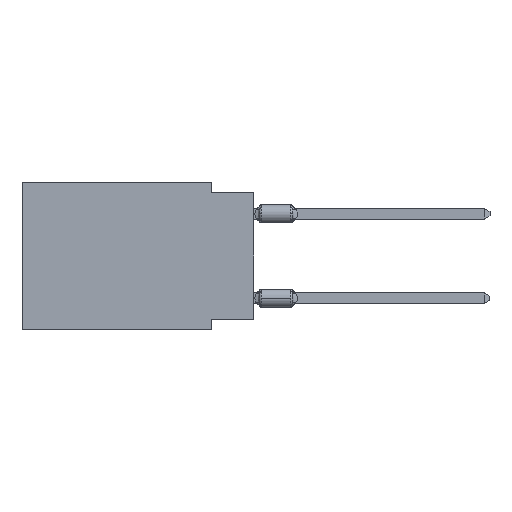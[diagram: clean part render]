
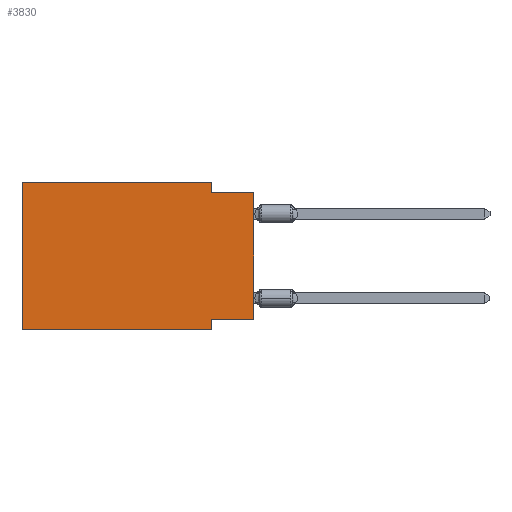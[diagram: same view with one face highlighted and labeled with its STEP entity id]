
A CAD part, left-side view. The second image highlights one B-rep face of the part: STEP entity #3830.
In plain terms, the highlighted planar face has unit normal (-1, 0, 0).
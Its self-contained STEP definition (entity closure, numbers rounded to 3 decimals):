
#281 = VERTEX_POINT ( 'NONE', #9532 ) ;
#521 = LINE ( 'NONE', #2627, #18176 ) ;
#1229 = ORIENTED_EDGE ( 'NONE', *, *, #23193, .F. ) ;
#1384 = DIRECTION ( 'NONE',  ( 0., 0., 1. ) ) ;
#1416 = EDGE_CURVE ( 'NONE', #16561, #22516, #3240, .T. ) ;
#1538 = FACE_OUTER_BOUND ( 'NONE', #6726, .T. ) ;
#2326 = ORIENTED_EDGE ( 'NONE', *, *, #19971, .F. ) ;
#2627 = CARTESIAN_POINT ( 'NONE',  ( 0., 2.54, 0. ) ) ;
#2996 = VECTOR ( 'NONE', #14350, 1000. ) ;
#3240 = LINE ( 'NONE', #9360, #22375 ) ;
#3404 = DIRECTION ( 'NONE',  ( 0., 0., -1. ) ) ;
#3830 = ADVANCED_FACE ( 'NONE', ( #1538 ), #9263, .F. ) ;
#4395 = LINE ( 'NONE', #23579, #9315 ) ;
#4775 = DIRECTION ( 'NONE',  ( 0., 1., 0. ) ) ;
#5116 = DIRECTION ( 'NONE',  ( 0., 0., 1. ) ) ;
#5329 = DIRECTION ( 'NONE',  ( 0., -1., 0. ) ) ;
#6117 = VERTEX_POINT ( 'NONE', #24452 ) ;
#6726 = EDGE_LOOP ( 'NONE', ( #11195, #1229, #22512, #2326, #14394, #18190, #17360, #9711 ) ) ;
#7140 = CARTESIAN_POINT ( 'NONE',  ( 0., 2.54, -0.635 ) ) ;
#7148 = EDGE_CURVE ( 'NONE', #281, #14565, #521, .T. ) ;
#7745 = EDGE_CURVE ( 'NONE', #16548, #15098, #13343, .T. ) ;
#8257 = CARTESIAN_POINT ( 'NONE',  ( 0., 13.97, 0. ) ) ;
#9263 = PLANE ( 'NONE',  #10916 ) ;
#9315 = VECTOR ( 'NONE', #4775, 1000. ) ;
#9360 = CARTESIAN_POINT ( 'NONE',  ( 0., 0., 0. ) ) ;
#9400 = LINE ( 'NONE', #17022, #20416 ) ;
#9532 = CARTESIAN_POINT ( 'NONE',  ( 0., 2.54, 0. ) ) ;
#9711 = ORIENTED_EDGE ( 'NONE', *, *, #21579, .F. ) ;
#9765 = DIRECTION ( 'NONE',  ( 0., 0., -1. ) ) ;
#10586 = CARTESIAN_POINT ( 'NONE',  ( 0., 13.97, 0. ) ) ;
#10916 = AXIS2_PLACEMENT_3D ( 'NONE', #24472, #18361, #3404 ) ;
#11195 = ORIENTED_EDGE ( 'NONE', *, *, #1416, .T. ) ;
#13343 = LINE ( 'NONE', #18704, #16519 ) ;
#14350 = DIRECTION ( 'NONE',  ( 0., -1., 0. ) ) ;
#14394 = ORIENTED_EDGE ( 'NONE', *, *, #14978, .F. ) ;
#14565 = VERTEX_POINT ( 'NONE', #7140 ) ;
#14978 = EDGE_CURVE ( 'NONE', #16548, #20276, #20056, .T. ) ;
#15098 = VERTEX_POINT ( 'NONE', #16836 ) ;
#15179 = LINE ( 'NONE', #20902, #24401 ) ;
#16100 = LINE ( 'NONE', #18072, #2996 ) ;
#16519 = VECTOR ( 'NONE', #21064, 1000. ) ;
#16548 = VERTEX_POINT ( 'NONE', #16711 ) ;
#16561 = VERTEX_POINT ( 'NONE', #24409 ) ;
#16711 = CARTESIAN_POINT ( 'NONE',  ( 0., 13.97, -8.89 ) ) ;
#16836 = CARTESIAN_POINT ( 'NONE',  ( 0., 2.54, -8.89 ) ) ;
#16936 = CARTESIAN_POINT ( 'NONE',  ( 0., 0., -0.635 ) ) ;
#17022 = CARTESIAN_POINT ( 'NONE',  ( 0., 2.54, -8.89 ) ) ;
#17360 = ORIENTED_EDGE ( 'NONE', *, *, #18734, .F. ) ;
#18072 = CARTESIAN_POINT ( 'NONE',  ( 0., 0., -0.635 ) ) ;
#18176 = VECTOR ( 'NONE', #21349, 1000. ) ;
#18190 = ORIENTED_EDGE ( 'NONE', *, *, #7745, .T. ) ;
#18361 = DIRECTION ( 'NONE',  ( 1., 0., 0. ) ) ;
#18704 = CARTESIAN_POINT ( 'NONE',  ( 0., 13.97, -8.89 ) ) ;
#18734 = EDGE_CURVE ( 'NONE', #6117, #15098, #9400, .T. ) ;
#19971 = EDGE_CURVE ( 'NONE', #20276, #281, #15179, .T. ) ;
#20056 = LINE ( 'NONE', #10586, #20825 ) ;
#20276 = VERTEX_POINT ( 'NONE', #8257 ) ;
#20416 = VECTOR ( 'NONE', #9765, 1000. ) ;
#20825 = VECTOR ( 'NONE', #5116, 1000. ) ;
#20902 = CARTESIAN_POINT ( 'NONE',  ( 0., 13.97, 0. ) ) ;
#21064 = DIRECTION ( 'NONE',  ( 0., -1., 0. ) ) ;
#21349 = DIRECTION ( 'NONE',  ( 0., 0., -1. ) ) ;
#21579 = EDGE_CURVE ( 'NONE', #16561, #6117, #4395, .T. ) ;
#22375 = VECTOR ( 'NONE', #1384, 1000. ) ;
#22512 = ORIENTED_EDGE ( 'NONE', *, *, #7148, .F. ) ;
#22516 = VERTEX_POINT ( 'NONE', #16936 ) ;
#23193 = EDGE_CURVE ( 'NONE', #14565, #22516, #16100, .T. ) ;
#23579 = CARTESIAN_POINT ( 'NONE',  ( 0., 0., -8.255 ) ) ;
#24401 = VECTOR ( 'NONE', #5329, 1000. ) ;
#24409 = CARTESIAN_POINT ( 'NONE',  ( 0., 0., -8.255 ) ) ;
#24452 = CARTESIAN_POINT ( 'NONE',  ( 0., 2.54, -8.255 ) ) ;
#24472 = CARTESIAN_POINT ( 'NONE',  ( 0., 13.97, 0. ) ) ;
